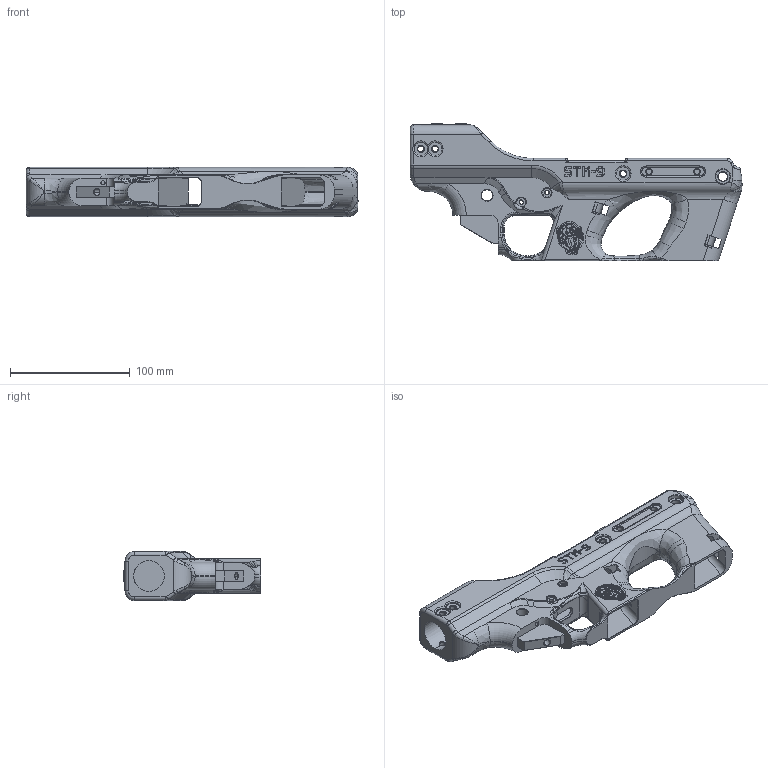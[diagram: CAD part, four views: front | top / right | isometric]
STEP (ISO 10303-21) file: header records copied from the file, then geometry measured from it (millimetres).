
FILE_DESCRIPTION (( 'STEP AP203' ), '1' );
FILE_NAME ('SaberToothMac-9-with-rail-mounts.STEP', '2022-03-10T01:01:06', ( '' ), ( '' ), 'SwSTEP 2.0', 'SolidWorks 2020', '' );
FILE_SCHEMA (( 'CONFIG_CONTROL_DESIGN' ));
Products named in the file (1): SaberToothMac-9-with-rail-mounts
Bounding box: 277 x 115.1 x 41 mm (x, y, z)
Volume: 311494.6 mm3; surface area: 99228 mm2
Topology: 1 solids, 1 shells, 2546 faces, 6664 edges, 4164 vertices
Faces by surface type: bspline 1089, plane 612, cylinder 548, torus 159, cone 106, sphere 32
Entity records: 117515 total; most frequent: CARTESIAN_POINT 62790, ORIENTED_EDGE 13184, DIRECTION 8433, EDGE_CURVE 6592, VERTEX_POINT 4157, AXIS2_PLACEMENT_3D 2834, VECTOR 2765, LINE 2765
